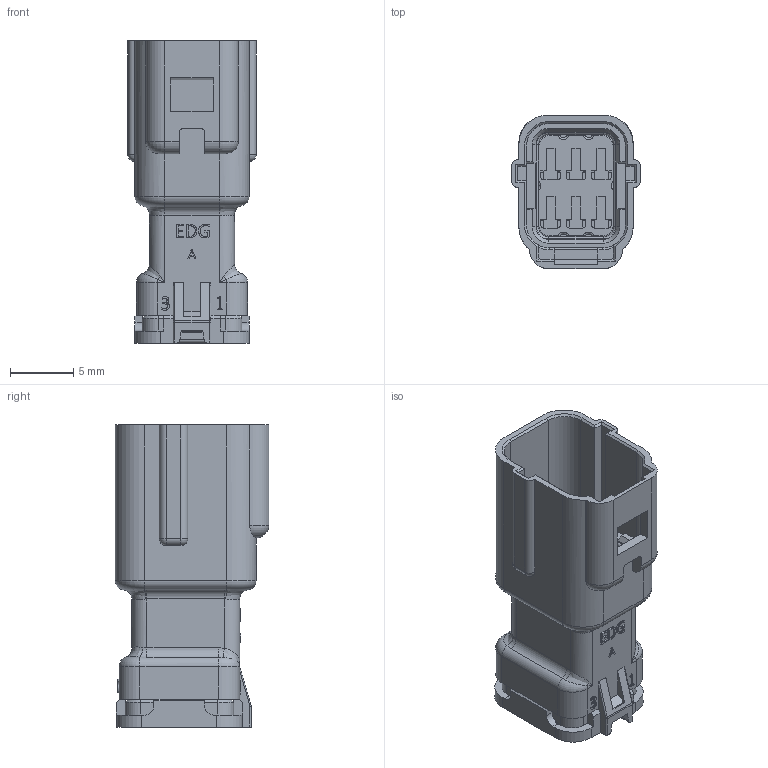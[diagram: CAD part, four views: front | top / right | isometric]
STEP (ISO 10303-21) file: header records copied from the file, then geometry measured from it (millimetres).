
FILE_DESCRIPTION (( 'STEP AP203' ), '1' );
FILE_NAME ('566-006-000-710.STEP', '2021-10-08T13:59:55', ( '' ), ( '' ), 'SwSTEP 2.0', 'SolidWorks 2020', '' );
FILE_SCHEMA (( 'CONFIG_CONTROL_DESIGN' ));
Length unit declared in the file: millimetre
Products named in the file (1): 566-006-000-710
Bounding box: 10.1 x 12.1 x 23.8 mm (x, y, z)
Volume: 1093.1 mm3; surface area: 2700.2 mm2
Topology: 2 solids, 11 shells, 1602 faces, 4138 edges, 2492 vertices
Faces by surface type: plane 769, cylinder 366, torus 305, cone 80, bspline 68, sphere 14
Entity records: 51615 total; most frequent: CARTESIAN_POINT 12655, ORIENTED_EDGE 8244, DIRECTION 8076, EDGE_CURVE 4122, AXIS2_PLACEMENT_3D 2739, LINE 2598, VECTOR 2598, VERTEX_POINT 2492
